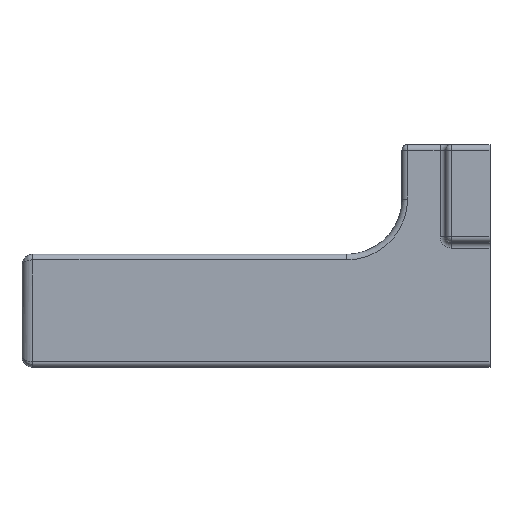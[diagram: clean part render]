
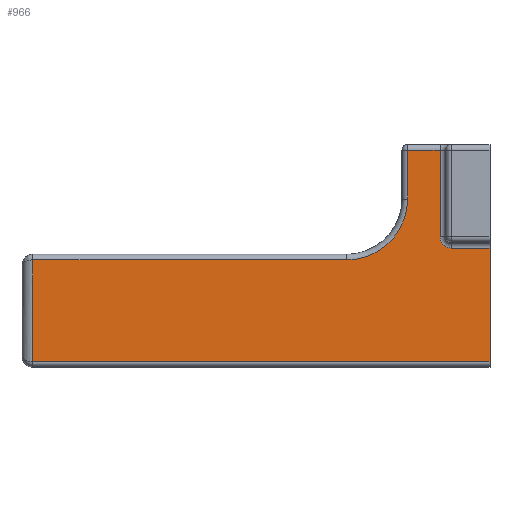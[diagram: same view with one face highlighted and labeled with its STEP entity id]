
A CAD part, top view. The second image highlights one B-rep face of the part: STEP entity #966.
In plain terms, the highlighted planar face has unit normal (0, 0, 1).
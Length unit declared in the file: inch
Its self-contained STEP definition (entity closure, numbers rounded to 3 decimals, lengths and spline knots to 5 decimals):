
#92=PLANE('',#1047);
#126=FACE_OUTER_BOUND('',#188,.T.);
#188=EDGE_LOOP('',(#745,#746,#747,#748,#749,#750,#751,#752,#753,#754));
#241=CIRCLE('',#1048,0.04);
#242=CIRCLE('',#1049,0.21685);
#280=LINE('',#1874,#327);
#281=LINE('',#2010,#328);
#283=LINE('',#2050,#330);
#284=LINE('',#2052,#331);
#285=LINE('',#2056,#332);
#286=LINE('',#2058,#333);
#287=LINE('',#2060,#334);
#288=LINE('',#2063,#335);
#327=VECTOR('',#1175,0.3937);
#328=VECTOR('',#1180,0.3937);
#330=VECTOR('',#1186,0.3937);
#331=VECTOR('',#1187,0.3937);
#332=VECTOR('',#1190,0.3937);
#333=VECTOR('',#1191,0.3937);
#334=VECTOR('',#1192,0.3937);
#335=VECTOR('',#1195,0.3937);
#419=VERTEX_POINT('',#1868);
#420=VERTEX_POINT('',#1872);
#427=VERTEX_POINT('',#2008);
#428=VERTEX_POINT('',#2049);
#429=VERTEX_POINT('',#2051);
#430=VERTEX_POINT('',#2053);
#431=VERTEX_POINT('',#2055);
#432=VERTEX_POINT('',#2057);
#433=VERTEX_POINT('',#2059);
#434=VERTEX_POINT('',#2061);
#525=EDGE_CURVE('',#420,#419,#280,.T.);
#539=EDGE_CURVE('',#427,#420,#281,.T.);
#542=EDGE_CURVE('',#427,#428,#283,.T.);
#543=EDGE_CURVE('',#429,#428,#284,.T.);
#544=EDGE_CURVE('',#430,#429,#241,.T.);
#545=EDGE_CURVE('',#431,#430,#285,.T.);
#546=EDGE_CURVE('',#432,#431,#286,.T.);
#547=EDGE_CURVE('',#433,#432,#287,.T.);
#548=EDGE_CURVE('',#434,#433,#242,.T.);
#549=EDGE_CURVE('',#419,#434,#288,.T.);
#745=ORIENTED_EDGE('',*,*,#539,.F.);
#746=ORIENTED_EDGE('',*,*,#542,.T.);
#747=ORIENTED_EDGE('',*,*,#543,.F.);
#748=ORIENTED_EDGE('',*,*,#544,.F.);
#749=ORIENTED_EDGE('',*,*,#545,.F.);
#750=ORIENTED_EDGE('',*,*,#546,.F.);
#751=ORIENTED_EDGE('',*,*,#547,.F.);
#752=ORIENTED_EDGE('',*,*,#548,.F.);
#753=ORIENTED_EDGE('',*,*,#549,.F.);
#754=ORIENTED_EDGE('',*,*,#525,.F.);
#966=ADVANCED_FACE('',(#126),#92,.T.);
#1047=AXIS2_PLACEMENT_3D('',#2048,#1184,#1185);
#1048=AXIS2_PLACEMENT_3D('',#2054,#1188,#1189);
#1049=AXIS2_PLACEMENT_3D('',#2062,#1193,#1194);
#1175=DIRECTION('',(0.,1.,0.));
#1180=DIRECTION('',(-1.,0.,0.));
#1184=DIRECTION('center_axis',(0.,0.,1.));
#1185=DIRECTION('ref_axis',(1.,0.,0.));
#1186=DIRECTION('',(0.,1.,0.));
#1187=DIRECTION('',(1.,0.,0.));
#1188=DIRECTION('center_axis',(0.,0.,1.));
#1189=DIRECTION('ref_axis',(-0.707,-0.707,0.));
#1190=DIRECTION('',(0.,-1.,0.));
#1191=DIRECTION('',(1.,0.,0.));
#1192=DIRECTION('',(0.,1.,0.));
#1193=DIRECTION('center_axis',(0.,0.,1.));
#1194=DIRECTION('ref_axis',(0.707,-0.707,0.));
#1195=DIRECTION('',(1.,0.,0.));
#1868=CARTESIAN_POINT('',(-1.6291,0.3826,0.3288));
#1872=CARTESIAN_POINT('',(-1.6291,0.02,0.3288));
#1874=CARTESIAN_POINT('',(-1.6291,0.39963,0.3288));
#2008=CARTESIAN_POINT('',(0.,0.02,0.3288));
#2010=CARTESIAN_POINT('',(-1.25138,0.02,0.3288));
#2048=CARTESIAN_POINT('Origin',(-0.83425,0.39665,0.3288));
#2049=CARTESIAN_POINT('',(0.,0.4249,0.3288));
#2050=CARTESIAN_POINT('',(0.,0.7933,0.3288));
#2051=CARTESIAN_POINT('',(-0.1378,0.4249,0.3288));
#2052=CARTESIAN_POINT('',(-0.49603,0.4249,0.3288));
#2053=CARTESIAN_POINT('',(-0.1778,0.4649,0.3288));
#2054=CARTESIAN_POINT('Origin',(-0.1378,0.4649,0.3288));
#2055=CARTESIAN_POINT('',(-0.1778,0.7733,0.3288));
#2056=CARTESIAN_POINT('',(-0.1778,0.59498,0.3288));
#2057=CARTESIAN_POINT('',(-0.2937,0.7733,0.3288));
#2058=CARTESIAN_POINT('',(-0.41713,0.7733,0.3288));
#2059=CARTESIAN_POINT('',(-0.2937,0.59945,0.3288));
#2060=CARTESIAN_POINT('',(-0.2937,0.59498,0.3288));
#2061=CARTESIAN_POINT('',(-0.51055,0.3826,0.3288));
#2062=CARTESIAN_POINT('Origin',(-0.51055,0.59945,0.3288));
#2063=CARTESIAN_POINT('',(-0.6724,0.3826,0.3288));
